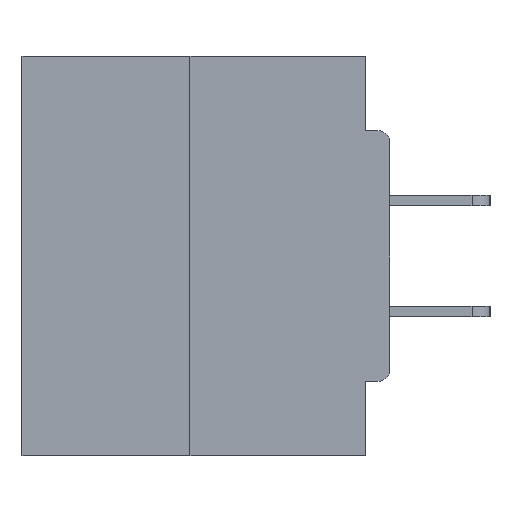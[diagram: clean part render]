
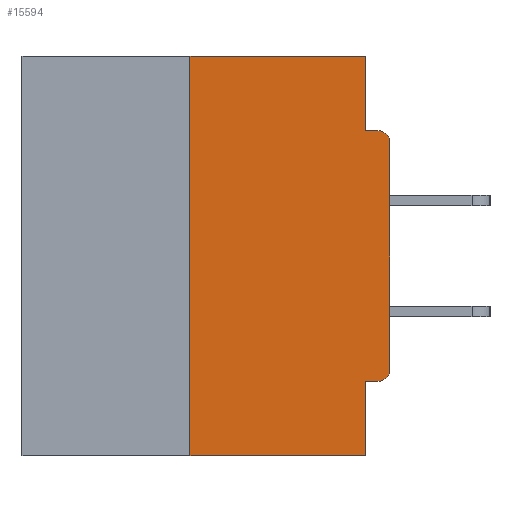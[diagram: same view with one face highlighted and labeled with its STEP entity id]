
A CAD part, left-side view. The second image highlights one B-rep face of the part: STEP entity #15594.
In plain terms, the highlighted planar face has unit normal (-1, 0, 0).
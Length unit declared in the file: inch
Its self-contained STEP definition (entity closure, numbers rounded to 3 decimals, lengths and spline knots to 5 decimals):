
#1008 = CARTESIAN_POINT ( 'NONE',  ( 0., 0.031, -0.4065 ) ) ;
#1038 = VERTEX_POINT ( 'NONE', #14754 ) ;
#2110 = LINE ( 'NONE', #6933, #7921 ) ;
#2959 = CARTESIAN_POINT ( 'NONE',  ( 0., 0.031, -0.0935 ) ) ;
#2958 = CARTESIAN_POINT ( 'NONE',  ( 0., 0.25, 0. ) ) ;
#3383 = VERTEX_POINT ( 'NONE', #2959 ) ;
#5002 = EDGE_CURVE ( 'NONE', #3383, #6947, #2110, .T. ) ;
#5263 = LINE ( 'NONE', #13357, #31733 ) ;
#5850 = ORIENTED_EDGE ( 'NONE', *, *, #27536, .T. ) ;
#5969 = EDGE_CURVE ( 'NONE', #12088, #11959, #13593, .T. ) ;
#6234 = DIRECTION ( 'NONE',  ( -1., 0., 0. ) ) ;
#6584 = CARTESIAN_POINT ( 'NONE',  ( 0., 0.46, -0.5 ) ) ;
#6632 = CARTESIAN_POINT ( 'NONE',  ( 0., 0.031, -0.5 ) ) ;
#6933 = CARTESIAN_POINT ( 'NONE',  ( 0., 0., -0.0935 ) ) ;
#6947 = VERTEX_POINT ( 'NONE', #9612 ) ;
#7042 = EDGE_LOOP ( 'NONE', ( #8192, #29182, #29086, #20622, #23335, #17648, #5850, #32435, #27078, #24724 ) ) ;
#7675 = LINE ( 'NONE', #28249, #33297 ) ;
#7921 = VECTOR ( 'NONE', #9480, 39.37008 ) ;
#8001 = EDGE_CURVE ( 'NONE', #33642, #30392, #8103, .T. ) ;
#8103 = LINE ( 'NONE', #6584, #13862 ) ;
#8192 = ORIENTED_EDGE ( 'NONE', *, *, #5969, .F. ) ;
#8287 = DIRECTION ( 'NONE',  ( 0., 0., 1. ) ) ;
#8863 = EDGE_CURVE ( 'NONE', #11959, #3383, #7675, .T. ) ;
#8899 = DIRECTION ( 'NONE',  ( 0., 0., -1. ) ) ;
#9387 = EDGE_CURVE ( 'NONE', #33642, #12088, #11951, .T. ) ;
#9457 = CARTESIAN_POINT ( 'NONE',  ( 0., 0.015, -0.3915 ) ) ;
#9480 = DIRECTION ( 'NONE',  ( 0., -1., 0. ) ) ;
#9612 = CARTESIAN_POINT ( 'NONE',  ( 0., 0.015, -0.0935 ) ) ;
#10379 = DIRECTION ( 'NONE',  ( 0., 0., -1. ) ) ;
#10482 = VECTOR ( 'NONE', #31099, 39.37008 ) ;
#11867 = CARTESIAN_POINT ( 'NONE',  ( 0., 0.015, -0.4065 ) ) ;
#11913 = AXIS2_PLACEMENT_3D ( 'NONE', #9457, #20044, #17610 ) ;
#11951 = LINE ( 'NONE', #2958, #33463 ) ;
#11959 = VERTEX_POINT ( 'NONE', #27865 ) ;
#12088 = VERTEX_POINT ( 'NONE', #33090 ) ;
#13003 = AXIS2_PLACEMENT_3D ( 'NONE', #14291, #6234, #8899 ) ;
#13250 = AXIS2_PLACEMENT_3D ( 'NONE', #31447, #17790, #20676 ) ;
#13357 = CARTESIAN_POINT ( 'NONE',  ( 0., 0.031, -0.5 ) ) ;
#13593 = LINE ( 'NONE', #24855, #32667 ) ;
#13775 = EDGE_CURVE ( 'NONE', #1038, #6947, #26930, .T. ) ;
#13847 = DIRECTION ( 'NONE',  ( 0., 1., 0. ) ) ;
#13862 = VECTOR ( 'NONE', #25048, 39.37008 ) ;
#14291 = CARTESIAN_POINT ( 'NONE',  ( 0., 0.015, -0.1085 ) ) ;
#14754 = CARTESIAN_POINT ( 'NONE',  ( 0., 0., -0.1085 ) ) ;
#15197 = VECTOR ( 'NONE', #13847, 39.37008 ) ;
#15594 = ADVANCED_FACE ( 'NONE', ( #23764 ), #20792, .F. ) ;
#15626 = LINE ( 'NONE', #16373, #15197 ) ;
#15893 = VERTEX_POINT ( 'NONE', #1008 ) ;
#16373 = CARTESIAN_POINT ( 'NONE',  ( 0., 0., -0.4065 ) ) ;
#17610 = DIRECTION ( 'NONE',  ( 0., 0., -1. ) ) ;
#17648 = ORIENTED_EDGE ( 'NONE', *, *, #24389, .T. ) ;
#17790 = DIRECTION ( 'NONE',  ( 1., 0., 0. ) ) ;
#18519 = CARTESIAN_POINT ( 'NONE',  ( 0., 0., -0.3915 ) ) ;
#19643 = DIRECTION ( 'NONE',  ( 0., -1., 0. ) ) ;
#20044 = DIRECTION ( 'NONE',  ( -1., 0., 0. ) ) ;
#20449 = VERTEX_POINT ( 'NONE', #18519 ) ;
#20622 = ORIENTED_EDGE ( 'NONE', *, *, #31603, .F. ) ;
#20676 = DIRECTION ( 'NONE',  ( 0., 0., -1. ) ) ;
#20792 = PLANE ( 'NONE',  #13250 ) ;
#23335 = ORIENTED_EDGE ( 'NONE', *, *, #24681, .F. ) ;
#23764 = FACE_OUTER_BOUND ( 'NONE', #7042, .T. ) ;
#24389 = EDGE_CURVE ( 'NONE', #30935, #20449, #31841, .T. ) ;
#24681 = EDGE_CURVE ( 'NONE', #30935, #15893, #15626, .T. ) ;
#24724 = ORIENTED_EDGE ( 'NONE', *, *, #8863, .F. ) ;
#24855 = CARTESIAN_POINT ( 'NONE',  ( 0., 0.46, 0. ) ) ;
#25048 = DIRECTION ( 'NONE',  ( 0., -1., 0. ) ) ;
#25410 = LINE ( 'NONE', #25435, #10482 ) ;
#25435 = CARTESIAN_POINT ( 'NONE',  ( 0., 0., 0. ) ) ;
#25687 = DIRECTION ( 'NONE',  ( 0., 0., -1. ) ) ;
#26930 = CIRCLE ( 'NONE', #13003, 0.015 ) ;
#27078 = ORIENTED_EDGE ( 'NONE', *, *, #5002, .F. ) ;
#27536 = EDGE_CURVE ( 'NONE', #20449, #1038, #25410, .T. ) ;
#27865 = CARTESIAN_POINT ( 'NONE',  ( 0., 0.031, 0. ) ) ;
#28249 = CARTESIAN_POINT ( 'NONE',  ( 0., 0.031, 0. ) ) ;
#28777 = CARTESIAN_POINT ( 'NONE',  ( 0., 0.25, -0.5 ) ) ;
#29086 = ORIENTED_EDGE ( 'NONE', *, *, #8001, .T. ) ;
#29182 = ORIENTED_EDGE ( 'NONE', *, *, #9387, .F. ) ;
#30392 = VERTEX_POINT ( 'NONE', #6632 ) ;
#30935 = VERTEX_POINT ( 'NONE', #11867 ) ;
#31099 = DIRECTION ( 'NONE',  ( 0., 0., 1. ) ) ;
#31447 = CARTESIAN_POINT ( 'NONE',  ( 0., 0.46, 0. ) ) ;
#31603 = EDGE_CURVE ( 'NONE', #15893, #30392, #5263, .T. ) ;
#31733 = VECTOR ( 'NONE', #10379, 39.37008 ) ;
#31841 = CIRCLE ( 'NONE', #11913, 0.015 ) ;
#32435 = ORIENTED_EDGE ( 'NONE', *, *, #13775, .T. ) ;
#32667 = VECTOR ( 'NONE', #19643, 39.37008 ) ;
#33090 = CARTESIAN_POINT ( 'NONE',  ( 0., 0.25, 0. ) ) ;
#33297 = VECTOR ( 'NONE', #25687, 39.37008 ) ;
#33463 = VECTOR ( 'NONE', #8287, 39.37008 ) ;
#33642 = VERTEX_POINT ( 'NONE', #28777 ) ;
